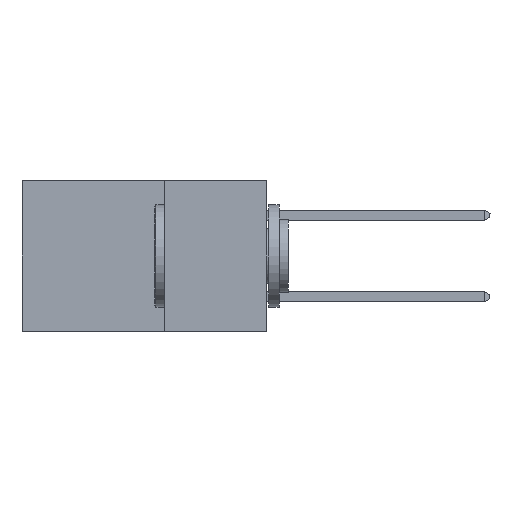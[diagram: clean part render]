
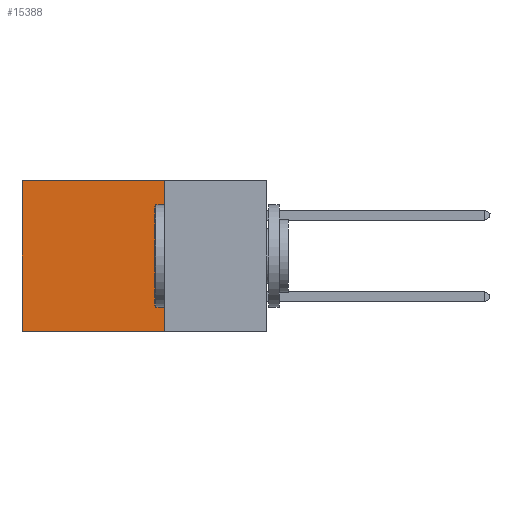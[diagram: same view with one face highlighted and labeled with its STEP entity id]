
A CAD part, left-side view. The second image highlights one B-rep face of the part: STEP entity #15388.
In plain terms, the highlighted planar face has unit normal (-1, 0, 0).
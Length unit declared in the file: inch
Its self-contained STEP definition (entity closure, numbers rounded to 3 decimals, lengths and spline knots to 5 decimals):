
#1332 = EDGE_CURVE ( 'NONE', #20640, #12819, #22476, .T. ) ;
#1565 = EDGE_CURVE ( 'NONE', #3570, #12819, #7521, .T. ) ;
#3570 = VERTEX_POINT ( 'NONE', #19836 ) ;
#3688 = CARTESIAN_POINT ( 'NONE',  ( 0.2875, 0.25, 0. ) ) ;
#5005 = CARTESIAN_POINT ( 'NONE',  ( 0.2875, 0.6, -0.37 ) ) ;
#7521 = LINE ( 'NONE', #15446, #11606 ) ;
#9548 = DIRECTION ( 'NONE',  ( 1., 0., 0. ) ) ;
#9847 = EDGE_CURVE ( 'NONE', #18139, #3570, #18016, .T. ) ;
#10571 = LINE ( 'NONE', #10896, #19440 ) ;
#10896 = CARTESIAN_POINT ( 'NONE',  ( 0.2875, 0.25, 0. ) ) ;
#11313 = AXIS2_PLACEMENT_3D ( 'NONE', #20148, #9548, #21952 ) ;
#11606 = VECTOR ( 'NONE', #13766, 39.37008 ) ;
#12669 = DIRECTION ( 'NONE',  ( 0., 1., 0. ) ) ;
#12819 = VERTEX_POINT ( 'NONE', #5005 ) ;
#13623 = ORIENTED_EDGE ( 'NONE', *, *, #1332, .T. ) ;
#13735 = ORIENTED_EDGE ( 'NONE', *, *, #21540, .T. ) ;
#13766 = DIRECTION ( 'NONE',  ( 0., 1., 0. ) ) ;
#14810 = PLANE ( 'NONE',  #11313 ) ;
#15388 = ADVANCED_FACE ( 'NONE', ( #20269 ), #14810, .F. ) ;
#15446 = CARTESIAN_POINT ( 'NONE',  ( 0.2875, 0.25, -0.37 ) ) ;
#15596 = CARTESIAN_POINT ( 'NONE',  ( 0.2875, 0.6, 0. ) ) ;
#15805 = ORIENTED_EDGE ( 'NONE', *, *, #9847, .F. ) ;
#15842 = EDGE_LOOP ( 'NONE', ( #13623, #16394, #15805, #13735 ) ) ;
#16083 = DIRECTION ( 'NONE',  ( 0., 0., -1. ) ) ;
#16394 = ORIENTED_EDGE ( 'NONE', *, *, #1565, .F. ) ;
#17090 = DIRECTION ( 'NONE',  ( 0., 0., -1. ) ) ;
#17312 = CARTESIAN_POINT ( 'NONE',  ( 0.2875, 0.6, 0. ) ) ;
#18016 = LINE ( 'NONE', #3688, #22209 ) ;
#18087 = CARTESIAN_POINT ( 'NONE',  ( 0.2875, 0.25, 0. ) ) ;
#18139 = VERTEX_POINT ( 'NONE', #18087 ) ;
#19440 = VECTOR ( 'NONE', #12669, 39.37008 ) ;
#19836 = CARTESIAN_POINT ( 'NONE',  ( 0.2875, 0.25, -0.37 ) ) ;
#20148 = CARTESIAN_POINT ( 'NONE',  ( 0.2875, 0.25, 0. ) ) ;
#20269 = FACE_OUTER_BOUND ( 'NONE', #15842, .T. ) ;
#20640 = VERTEX_POINT ( 'NONE', #15596 ) ;
#21372 = VECTOR ( 'NONE', #17090, 39.37008 ) ;
#21540 = EDGE_CURVE ( 'NONE', #18139, #20640, #10571, .T. ) ;
#21952 = DIRECTION ( 'NONE',  ( 0., 0., -1. ) ) ;
#22209 = VECTOR ( 'NONE', #16083, 39.37008 ) ;
#22476 = LINE ( 'NONE', #17312, #21372 ) ;
